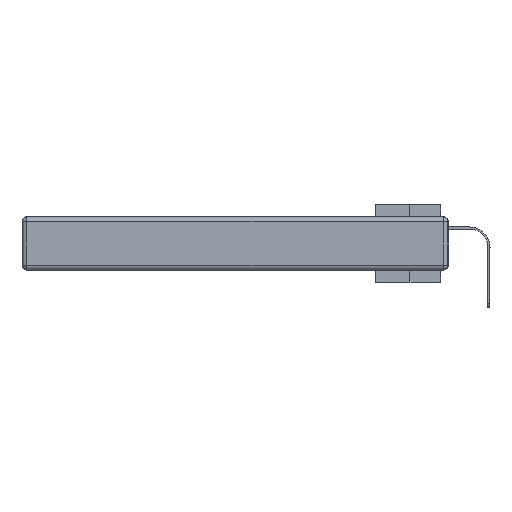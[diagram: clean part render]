
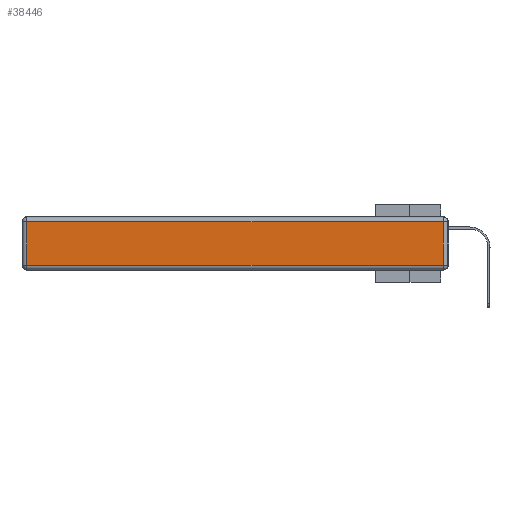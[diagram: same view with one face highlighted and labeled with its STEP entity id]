
A CAD part, left-side view. The second image highlights one B-rep face of the part: STEP entity #38446.
In plain terms, the highlighted planar face has unit normal (-1, 0, 0).
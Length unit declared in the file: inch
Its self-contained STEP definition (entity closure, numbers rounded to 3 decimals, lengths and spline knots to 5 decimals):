
#2373 = VECTOR ( 'NONE', #35615, 39.37008 ) ;
#3621 = VECTOR ( 'NONE', #25947, 39.37008 ) ;
#3795 = DIRECTION ( 'NONE',  ( 0., 0., -1. ) ) ;
#4711 = CARTESIAN_POINT ( 'NONE',  ( 0., 0.03, -0.03 ) ) ;
#4901 = VERTEX_POINT ( 'NONE', #5422 ) ;
#5422 = CARTESIAN_POINT ( 'NONE',  ( 0., 0.03, -0.313 ) ) ;
#7109 = ORIENTED_EDGE ( 'NONE', *, *, #19211, .T. ) ;
#7311 = LINE ( 'NONE', #28350, #3621 ) ;
#9016 = PLANE ( 'NONE',  #22512 ) ;
#11017 = VECTOR ( 'NONE', #3795, 39.37008 ) ;
#13649 = ORIENTED_EDGE ( 'NONE', *, *, #15898, .T. ) ;
#14171 = VERTEX_POINT ( 'NONE', #25903 ) ;
#15211 = DIRECTION ( 'NONE',  ( 0., 0., 1. ) ) ;
#15898 = EDGE_CURVE ( 'NONE', #31028, #20585, #20986, .T. ) ;
#17894 = ORIENTED_EDGE ( 'NONE', *, *, #21833, .T. ) ;
#18228 = LINE ( 'NONE', #24852, #11017 ) ;
#19211 = EDGE_CURVE ( 'NONE', #4901, #31028, #7311, .T. ) ;
#20369 = CARTESIAN_POINT ( 'NONE',  ( 0., 2.72, -0.03 ) ) ;
#20585 = VERTEX_POINT ( 'NONE', #20369 ) ;
#20986 = LINE ( 'NONE', #30203, #23321 ) ;
#21239 = FACE_OUTER_BOUND ( 'NONE', #33189, .T. ) ;
#21627 = DIRECTION ( 'NONE',  ( -1., 0., 0. ) ) ;
#21833 = EDGE_CURVE ( 'NONE', #14171, #4901, #23000, .T. ) ;
#22512 = AXIS2_PLACEMENT_3D ( 'NONE', #27046, #21627, #15211 ) ;
#23000 = LINE ( 'NONE', #25806, #2373 ) ;
#23321 = VECTOR ( 'NONE', #27396, 39.37008 ) ;
#24852 = CARTESIAN_POINT ( 'NONE',  ( 0., 2.72, -0.343 ) ) ;
#25806 = CARTESIAN_POINT ( 'NONE',  ( 0., 0., -0.313 ) ) ;
#25903 = CARTESIAN_POINT ( 'NONE',  ( 0., 2.72, -0.313 ) ) ;
#25947 = DIRECTION ( 'NONE',  ( 0., 0., 1. ) ) ;
#27046 = CARTESIAN_POINT ( 'NONE',  ( 0., 0., -0.343 ) ) ;
#27396 = DIRECTION ( 'NONE',  ( 0., 1., 0. ) ) ;
#27693 = ORIENTED_EDGE ( 'NONE', *, *, #29981, .T. ) ;
#28350 = CARTESIAN_POINT ( 'NONE',  ( 0., 0.03, -0.343 ) ) ;
#29981 = EDGE_CURVE ( 'NONE', #20585, #14171, #18228, .T. ) ;
#30203 = CARTESIAN_POINT ( 'NONE',  ( 0., 2.75, -0.03 ) ) ;
#31028 = VERTEX_POINT ( 'NONE', #4711 ) ;
#33189 = EDGE_LOOP ( 'NONE', ( #17894, #7109, #13649, #27693 ) ) ;
#35615 = DIRECTION ( 'NONE',  ( 0., -1., 0. ) ) ;
#38446 = ADVANCED_FACE ( 'NONE', ( #21239 ), #9016, .T. ) ;
